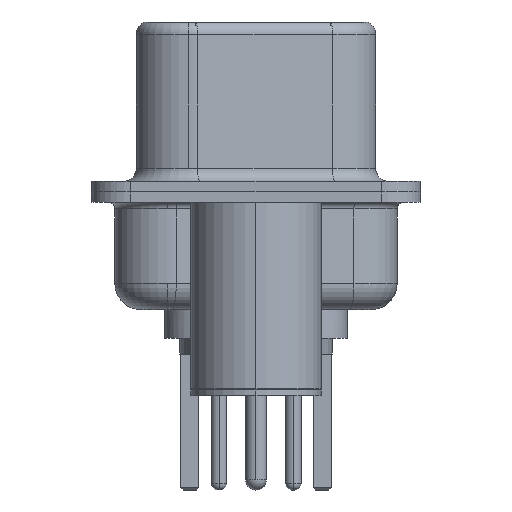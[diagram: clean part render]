
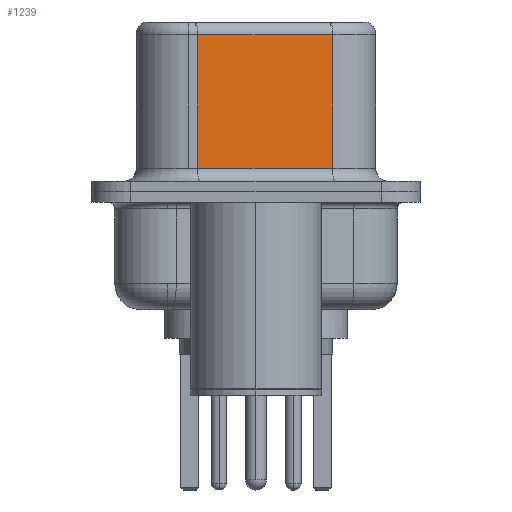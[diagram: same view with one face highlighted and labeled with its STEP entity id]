
A CAD part, left-side view. The second image highlights one B-rep face of the part: STEP entity #1239.
In plain terms, the highlighted planar face has unit normal (-0.985, -0.174, 0).
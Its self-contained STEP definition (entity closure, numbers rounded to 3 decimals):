
#1239 = ADVANCED_FACE ( 'NONE', ( #16218 ), #25416, .F. ) ;
#1394 = DIRECTION ( 'NONE',  ( 0., 0., -1. ) ) ;
#2294 = ORIENTED_EDGE ( 'NONE', *, *, #24666, .T. ) ;
#2447 = VECTOR ( 'NONE', #17368, 1000. ) ;
#4652 = LINE ( 'NONE', #23994, #14881 ) ;
#5188 = CARTESIAN_POINT ( 'NONE',  ( 4.58, -2.927, 6.02 ) ) ;
#5227 = EDGE_LOOP ( 'NONE', ( #12520, #5699, #25086, #2294 ) ) ;
#5699 = ORIENTED_EDGE ( 'NONE', *, *, #24544, .T. ) ;
#5712 = CARTESIAN_POINT ( 'NONE',  ( 3.67, 2.233, 6.52 ) ) ;
#5912 = VERTEX_POINT ( 'NONE', #8417 ) ;
#6595 = LINE ( 'NONE', #11509, #16828 ) ;
#7234 = CARTESIAN_POINT ( 'NONE',  ( 3.67, 2.233, 6.02 ) ) ;
#7737 = AXIS2_PLACEMENT_3D ( 'NONE', #24762, #23262, #23234 ) ;
#8417 = CARTESIAN_POINT ( 'NONE',  ( 3.67, 2.233, 0.9 ) ) ;
#9759 = DIRECTION ( 'NONE',  ( 0., 0., -1. ) ) ;
#9864 = EDGE_CURVE ( 'NONE', #25220, #5912, #13332, .T. ) ;
#10689 = VERTEX_POINT ( 'NONE', #17394 ) ;
#11509 = CARTESIAN_POINT ( 'NONE',  ( 4.58, -2.927, 6.52 ) ) ;
#12520 = ORIENTED_EDGE ( 'NONE', *, *, #22617, .F. ) ;
#13298 = LINE ( 'NONE', #5188, #2447 ) ;
#13332 = LINE ( 'NONE', #5712, #22905 ) ;
#14881 = VECTOR ( 'NONE', #26062, 1000. ) ;
#16218 = FACE_OUTER_BOUND ( 'NONE', #5227, .T. ) ;
#16828 = VECTOR ( 'NONE', #1394, 1000. ) ;
#17368 = DIRECTION ( 'NONE',  ( -0.174, 0.985, 0. ) ) ;
#17394 = CARTESIAN_POINT ( 'NONE',  ( 4.58, -2.927, 0.9 ) ) ;
#18596 = VERTEX_POINT ( 'NONE', #22722 ) ;
#22617 = EDGE_CURVE ( 'NONE', #18596, #10689, #6595, .T. ) ;
#22722 = CARTESIAN_POINT ( 'NONE',  ( 4.58, -2.927, 6.02 ) ) ;
#22905 = VECTOR ( 'NONE', #9759, 1000. ) ;
#23234 = DIRECTION ( 'NONE',  ( -0.174, 0.985, 0. ) ) ;
#23262 = DIRECTION ( 'NONE',  ( 0.985, 0.174, 0. ) ) ;
#23994 = CARTESIAN_POINT ( 'NONE',  ( 4.58, -2.927, 0.9 ) ) ;
#24544 = EDGE_CURVE ( 'NONE', #18596, #25220, #13298, .T. ) ;
#24666 = EDGE_CURVE ( 'NONE', #5912, #10689, #4652, .T. ) ;
#24762 = CARTESIAN_POINT ( 'NONE',  ( 4.58, -2.927, 6.52 ) ) ;
#25086 = ORIENTED_EDGE ( 'NONE', *, *, #9864, .T. ) ;
#25220 = VERTEX_POINT ( 'NONE', #7234 ) ;
#25416 = PLANE ( 'NONE',  #7737 ) ;
#26062 = DIRECTION ( 'NONE',  ( 0.174, -0.985, 0. ) ) ;
